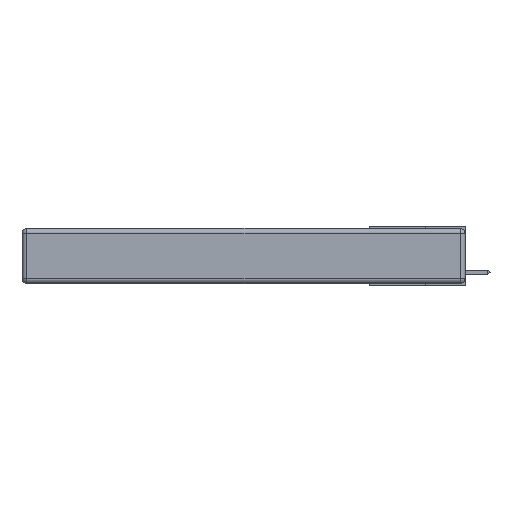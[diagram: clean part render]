
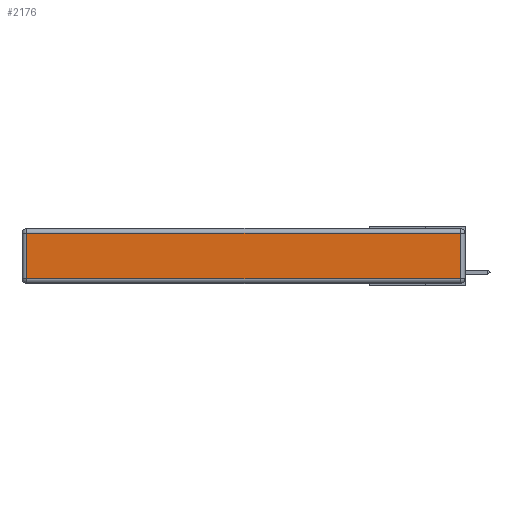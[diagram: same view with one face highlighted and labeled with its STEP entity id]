
A CAD part, left-side view. The second image highlights one B-rep face of the part: STEP entity #2176.
In plain terms, the highlighted planar face has unit normal (-1, 0, 0).
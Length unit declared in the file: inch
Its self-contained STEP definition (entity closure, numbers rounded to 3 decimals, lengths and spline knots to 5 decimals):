
#548 = VECTOR ( 'NONE', #8666, 39.37008 ) ;
#1302 = LINE ( 'NONE', #10389, #6580 ) ;
#1318 = CARTESIAN_POINT ( 'NONE',  ( 0., 0., -0.343 ) ) ;
#1406 = ORIENTED_EDGE ( 'NONE', *, *, #4654, .T. ) ;
#1767 = DIRECTION ( 'NONE',  ( -1., 0., 0. ) ) ;
#2176 = ADVANCED_FACE ( 'NONE', ( #15560 ), #10205, .T. ) ;
#2779 = CARTESIAN_POINT ( 'NONE',  ( 0., 2.72, -0.313 ) ) ;
#3000 = DIRECTION ( 'NONE',  ( 0., 0., 1. ) ) ;
#3027 = EDGE_LOOP ( 'NONE', ( #4350, #1406, #12733, #6378 ) ) ;
#3439 = EDGE_CURVE ( 'NONE', #7909, #15087, #5995, .T. ) ;
#3530 = CARTESIAN_POINT ( 'NONE',  ( 0., 0.03, -0.03 ) ) ;
#3843 = VECTOR ( 'NONE', #14277, 39.37008 ) ;
#4235 = EDGE_CURVE ( 'NONE', #13822, #8527, #8326, .T. ) ;
#4350 = ORIENTED_EDGE ( 'NONE', *, *, #3439, .T. ) ;
#4654 = EDGE_CURVE ( 'NONE', #15087, #13822, #1302, .T. ) ;
#5183 = CARTESIAN_POINT ( 'NONE',  ( 0., 0.03, -0.313 ) ) ;
#5995 = LINE ( 'NONE', #8779, #548 ) ;
#6223 = DIRECTION ( 'NONE',  ( 0., 0., -1. ) ) ;
#6378 = ORIENTED_EDGE ( 'NONE', *, *, #11803, .T. ) ;
#6580 = VECTOR ( 'NONE', #15269, 39.37008 ) ;
#6738 = AXIS2_PLACEMENT_3D ( 'NONE', #1318, #1767, #3000 ) ;
#7588 = VECTOR ( 'NONE', #6223, 39.37008 ) ;
#7909 = VERTEX_POINT ( 'NONE', #2779 ) ;
#8326 = LINE ( 'NONE', #9943, #3843 ) ;
#8527 = VERTEX_POINT ( 'NONE', #13163 ) ;
#8666 = DIRECTION ( 'NONE',  ( 0., -1., 0. ) ) ;
#8779 = CARTESIAN_POINT ( 'NONE',  ( 0., 0., -0.313 ) ) ;
#9943 = CARTESIAN_POINT ( 'NONE',  ( 0., 2.75, -0.03 ) ) ;
#10205 = PLANE ( 'NONE',  #6738 ) ;
#10389 = CARTESIAN_POINT ( 'NONE',  ( 0., 0.03, -0.343 ) ) ;
#10923 = LINE ( 'NONE', #11279, #7588 ) ;
#11279 = CARTESIAN_POINT ( 'NONE',  ( 0., 2.72, -0.343 ) ) ;
#11803 = EDGE_CURVE ( 'NONE', #8527, #7909, #10923, .T. ) ;
#12733 = ORIENTED_EDGE ( 'NONE', *, *, #4235, .T. ) ;
#13163 = CARTESIAN_POINT ( 'NONE',  ( 0., 2.72, -0.03 ) ) ;
#13822 = VERTEX_POINT ( 'NONE', #3530 ) ;
#14277 = DIRECTION ( 'NONE',  ( 0., 1., 0. ) ) ;
#15087 = VERTEX_POINT ( 'NONE', #5183 ) ;
#15269 = DIRECTION ( 'NONE',  ( 0., 0., 1. ) ) ;
#15560 = FACE_OUTER_BOUND ( 'NONE', #3027, .T. ) ;
